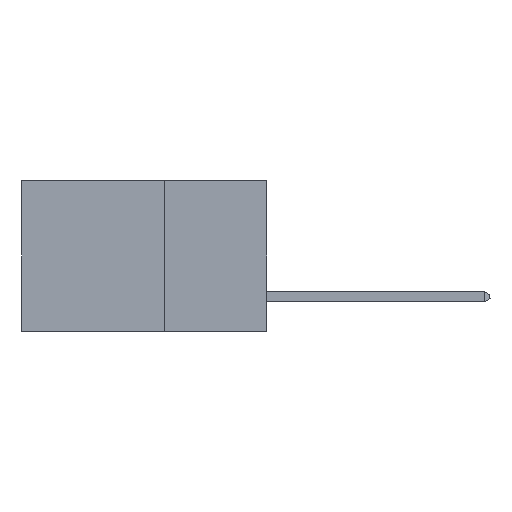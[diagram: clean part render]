
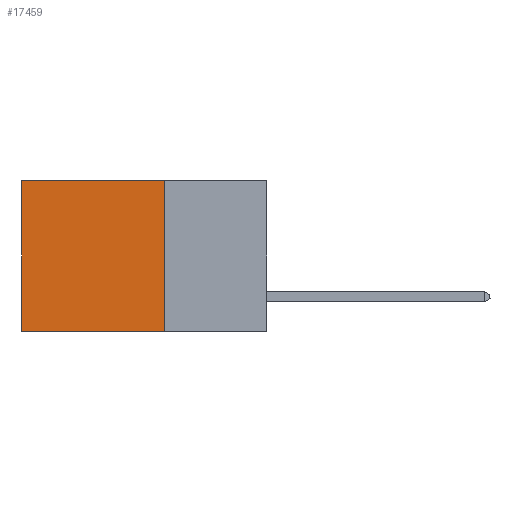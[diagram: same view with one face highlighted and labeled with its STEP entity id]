
A CAD part, left-side view. The second image highlights one B-rep face of the part: STEP entity #17459.
In plain terms, the highlighted planar face has unit normal (-1, 0, 0).
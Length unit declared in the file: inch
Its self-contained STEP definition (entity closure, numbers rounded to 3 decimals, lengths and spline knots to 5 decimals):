
#763 = VERTEX_POINT ( 'NONE', #3862 ) ;
#838 = CARTESIAN_POINT ( 'NONE',  ( 0.2875, 0.6, 0. ) ) ;
#878 = LINE ( 'NONE', #4696, #11083 ) ;
#910 = DIRECTION ( 'NONE',  ( 1., 0., 0. ) ) ;
#1081 = EDGE_LOOP ( 'NONE', ( #3121, #12683, #2369, #12856 ) ) ;
#2148 = LINE ( 'NONE', #14499, #6504 ) ;
#2369 = ORIENTED_EDGE ( 'NONE', *, *, #19948, .F. ) ;
#2651 = VERTEX_POINT ( 'NONE', #838 ) ;
#3121 = ORIENTED_EDGE ( 'NONE', *, *, #4619, .T. ) ;
#3335 = VECTOR ( 'NONE', #9692, 39.37008 ) ;
#3862 = CARTESIAN_POINT ( 'NONE',  ( 0.2875, 0.6, -0.37 ) ) ;
#4619 = EDGE_CURVE ( 'NONE', #2651, #763, #2148, .T. ) ;
#4660 = EDGE_CURVE ( 'NONE', #14871, #763, #19685, .T. ) ;
#4696 = CARTESIAN_POINT ( 'NONE',  ( 0.2875, 0.25, 0. ) ) ;
#6504 = VECTOR ( 'NONE', #14725, 39.37008 ) ;
#6519 = DIRECTION ( 'NONE',  ( 0., 1., 0. ) ) ;
#7371 = EDGE_CURVE ( 'NONE', #15409, #2651, #16792, .T. ) ;
#8368 = FACE_OUTER_BOUND ( 'NONE', #1081, .T. ) ;
#9647 = CARTESIAN_POINT ( 'NONE',  ( 0.2875, 0.25, 0. ) ) ;
#9692 = DIRECTION ( 'NONE',  ( 0., 1., 0. ) ) ;
#9808 = VECTOR ( 'NONE', #6519, 39.37008 ) ;
#10828 = PLANE ( 'NONE',  #12106 ) ;
#11083 = VECTOR ( 'NONE', #17422, 39.37008 ) ;
#11312 = CARTESIAN_POINT ( 'NONE',  ( 0.2875, 0.25, 0. ) ) ;
#12106 = AXIS2_PLACEMENT_3D ( 'NONE', #12423, #910, #17381 ) ;
#12423 = CARTESIAN_POINT ( 'NONE',  ( 0.2875, 0.25, 0. ) ) ;
#12683 = ORIENTED_EDGE ( 'NONE', *, *, #4660, .F. ) ;
#12856 = ORIENTED_EDGE ( 'NONE', *, *, #7371, .T. ) ;
#14499 = CARTESIAN_POINT ( 'NONE',  ( 0.2875, 0.6, 0. ) ) ;
#14725 = DIRECTION ( 'NONE',  ( 0., 0., -1. ) ) ;
#14871 = VERTEX_POINT ( 'NONE', #18307 ) ;
#15409 = VERTEX_POINT ( 'NONE', #9647 ) ;
#16209 = CARTESIAN_POINT ( 'NONE',  ( 0.2875, 0.25, -0.37 ) ) ;
#16792 = LINE ( 'NONE', #11312, #3335 ) ;
#17381 = DIRECTION ( 'NONE',  ( 0., 0., -1. ) ) ;
#17422 = DIRECTION ( 'NONE',  ( 0., 0., -1. ) ) ;
#17459 = ADVANCED_FACE ( 'NONE', ( #8368 ), #10828, .F. ) ;
#18307 = CARTESIAN_POINT ( 'NONE',  ( 0.2875, 0.25, -0.37 ) ) ;
#19685 = LINE ( 'NONE', #16209, #9808 ) ;
#19948 = EDGE_CURVE ( 'NONE', #15409, #14871, #878, .T. ) ;
